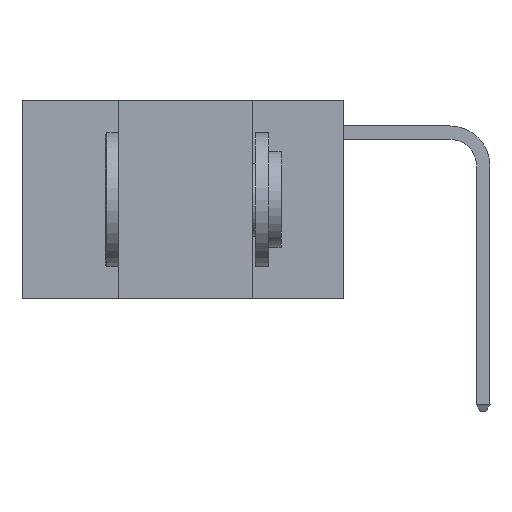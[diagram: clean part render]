
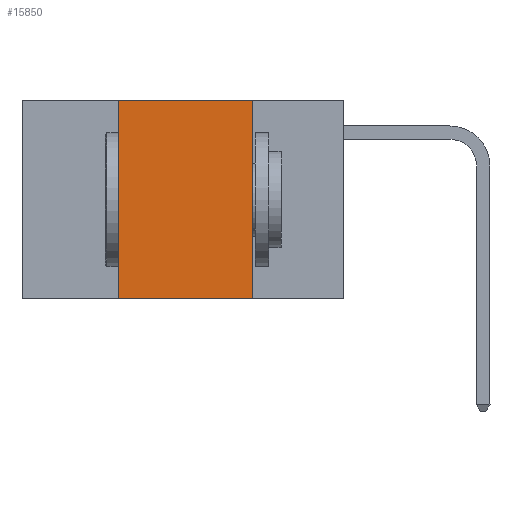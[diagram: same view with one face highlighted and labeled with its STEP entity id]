
A CAD part, left-side view. The second image highlights one B-rep face of the part: STEP entity #15850.
In plain terms, the highlighted planar face has unit normal (-1, 0, 0).
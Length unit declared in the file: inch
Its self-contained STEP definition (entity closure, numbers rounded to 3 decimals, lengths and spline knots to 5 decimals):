
#17 = VERTEX_POINT ( 'NONE', #12051 ) ;
#324 = FACE_OUTER_BOUND ( 'NONE', #398, .T. ) ;
#398 = EDGE_LOOP ( 'NONE', ( #14847, #8583, #15203, #8973 ) ) ;
#1343 = LINE ( 'NONE', #12101, #10669 ) ;
#1606 = LINE ( 'NONE', #1916, #13873 ) ;
#1916 = CARTESIAN_POINT ( 'NONE',  ( 0., 0.42, 0. ) ) ;
#2475 = CARTESIAN_POINT ( 'NONE',  ( 0., 0.17, 0. ) ) ;
#2480 = EDGE_CURVE ( 'NONE', #9368, #13141, #12313, .T. ) ;
#3041 = DIRECTION ( 'NONE',  ( 0., 0., -1. ) ) ;
#3069 = LINE ( 'NONE', #16010, #13148 ) ;
#4134 = CARTESIAN_POINT ( 'NONE',  ( 0., 0.17, 0. ) ) ;
#4976 = PLANE ( 'NONE',  #6739 ) ;
#5706 = CARTESIAN_POINT ( 'NONE',  ( 0., 0.17, -0.37 ) ) ;
#6739 = AXIS2_PLACEMENT_3D ( 'NONE', #7527, #16187, #8779 ) ;
#6841 = EDGE_CURVE ( 'NONE', #17, #11199, #1606, .T. ) ;
#7527 = CARTESIAN_POINT ( 'NONE',  ( 0., 0.6, 0. ) ) ;
#8583 = ORIENTED_EDGE ( 'NONE', *, *, #12147, .F. ) ;
#8779 = DIRECTION ( 'NONE',  ( 0., 0., -1. ) ) ;
#8973 = ORIENTED_EDGE ( 'NONE', *, *, #16249, .T. ) ;
#9368 = VERTEX_POINT ( 'NONE', #4134 ) ;
#9498 = DIRECTION ( 'NONE',  ( 0., 0., 1. ) ) ;
#9862 = DIRECTION ( 'NONE',  ( 0., -1., 0. ) ) ;
#10669 = VECTOR ( 'NONE', #13344, 39.37008 ) ;
#11199 = VERTEX_POINT ( 'NONE', #15362 ) ;
#12051 = CARTESIAN_POINT ( 'NONE',  ( 0., 0.42, -0.37 ) ) ;
#12101 = CARTESIAN_POINT ( 'NONE',  ( 0., 0.6, -0.37 ) ) ;
#12147 = EDGE_CURVE ( 'NONE', #11199, #9368, #3069, .T. ) ;
#12313 = LINE ( 'NONE', #2475, #15903 ) ;
#13141 = VERTEX_POINT ( 'NONE', #5706 ) ;
#13148 = VECTOR ( 'NONE', #9862, 39.37008 ) ;
#13344 = DIRECTION ( 'NONE',  ( 0., -1., 0. ) ) ;
#13873 = VECTOR ( 'NONE', #9498, 39.37008 ) ;
#14847 = ORIENTED_EDGE ( 'NONE', *, *, #2480, .F. ) ;
#15203 = ORIENTED_EDGE ( 'NONE', *, *, #6841, .F. ) ;
#15362 = CARTESIAN_POINT ( 'NONE',  ( 0., 0.42, 0. ) ) ;
#15850 = ADVANCED_FACE ( 'NONE', ( #324 ), #4976, .F. ) ;
#15903 = VECTOR ( 'NONE', #3041, 39.37008 ) ;
#16010 = CARTESIAN_POINT ( 'NONE',  ( 0., 0.6, 0. ) ) ;
#16187 = DIRECTION ( 'NONE',  ( 1., 0., 0. ) ) ;
#16249 = EDGE_CURVE ( 'NONE', #17, #13141, #1343, .T. ) ;
